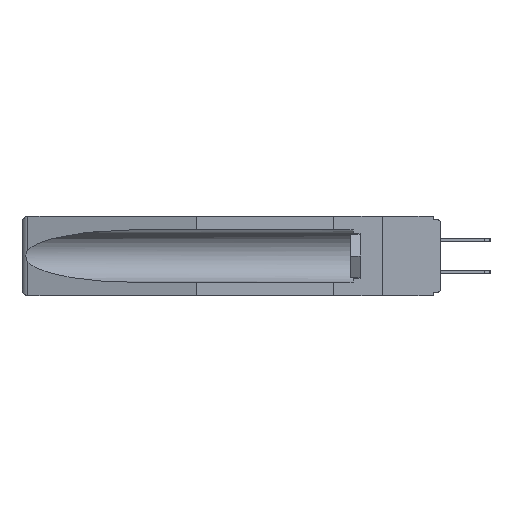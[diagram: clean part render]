
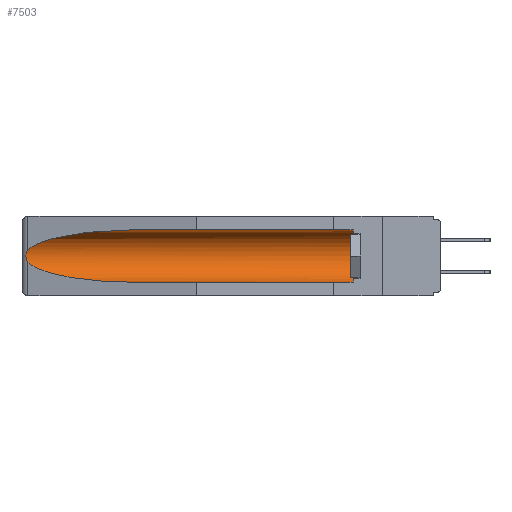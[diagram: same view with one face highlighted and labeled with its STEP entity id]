
A CAD part, left-side view. The second image highlights one B-rep face of the part: STEP entity #7503.
In plain terms, the highlighted cylindrical face has radius 2.857 mm (diameter 5.715 mm), a partial arc.
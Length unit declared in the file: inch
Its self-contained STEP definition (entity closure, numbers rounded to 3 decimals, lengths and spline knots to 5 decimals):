
#12 = CARTESIAN_POINT ( 'NONE',  ( 0.21114, 1.30732, -0.284 ) ) ;
#1002 = EDGE_LOOP ( 'NONE', ( #23991, #11615, #4133, #8195, #10715, #6035 ) ) ;
#1873 = AXIS2_PLACEMENT_3D ( 'NONE', #24452, #8560, #10771 ) ;
#2198 = CARTESIAN_POINT ( 'NONE',  ( 0.26597, 1.52961, -0.15275 ) ) ;
#2941 = CARTESIAN_POINT ( 'NONE',  ( 0.155, -0.30754, -0.284 ) ) ;
#4027 = VERTEX_POINT ( 'NONE', #26024 ) ;
#4091 = CARTESIAN_POINT ( 'NONE',  ( 0.155, 0.126, -0.284 ) ) ;
#4133 = ORIENTED_EDGE ( 'NONE', *, *, #19639, .T. ) ;
#5881 =( BOUNDED_CURVE ( )  B_SPLINE_CURVE ( 3, ( #20720, #25322, #7179, #11658 ),
 .UNSPECIFIED., .F., .F. ) 
 B_SPLINE_CURVE_WITH_KNOTS ( ( 4, 4 ),
 ( 4.71239, 6.08839 ),
 .UNSPECIFIED. ) 
 CURVE ( )  GEOMETRIC_REPRESENTATION_ITEM ( )  RATIONAL_B_SPLINE_CURVE ( ( 1., 0.848, 0.848, 1. ) ) 
 REPRESENTATION_ITEM ( '' )  );
#6035 = ORIENTED_EDGE ( 'NONE', *, *, #18235, .T. ) ;
#6184 = CARTESIAN_POINT ( 'NONE',  ( 0.155, 1.07973, -0.059 ) ) ;
#6787 = VERTEX_POINT ( 'NONE', #13449 ) ;
#6799 = CARTESIAN_POINT ( 'NONE',  ( 0.2675, 1.53308, -0.17534 ) ) ;
#6876 = LINE ( 'NONE', #10090, #29344 ) ;
#6960 = CIRCLE ( 'NONE', #1873, 0.1125 ) ;
#7024 = EDGE_CURVE ( 'NONE', #7655, #4027, #5881, .T. ) ;
#7094 = CARTESIAN_POINT ( 'NONE',  ( 0.26597, 1.5296, -0.19026 ) ) ;
#7179 = CARTESIAN_POINT ( 'NONE',  ( 0.25451, 1.48313, -0.09465 ) ) ;
#7503 = ADVANCED_FACE ( 'NONE', ( #28855 ), #17768, .F. ) ;
#7655 = VERTEX_POINT ( 'NONE', #6184 ) ;
#8195 = ORIENTED_EDGE ( 'NONE', *, *, #24356, .F. ) ;
#8560 = DIRECTION ( 'NONE',  ( 0., -1., 0. ) ) ;
#9345 = CARTESIAN_POINT ( 'NONE',  ( 0.26655, 1.53094, -0.18657 ) ) ;
#9802 = VERTEX_POINT ( 'NONE', #21206 ) ;
#10063 = VERTEX_POINT ( 'NONE', #24503 ) ;
#10090 = CARTESIAN_POINT ( 'NONE',  ( 0.155, -0.30754, -0.059 ) ) ;
#10715 = ORIENTED_EDGE ( 'NONE', *, *, #17072, .T. ) ;
#10771 = DIRECTION ( 'NONE',  ( 0., 0., 1. ) ) ;
#11158 = B_SPLINE_CURVE_WITH_KNOTS ( 'NONE', 3,
 ( #11564, #2198, #24940, #22628, #18446, #6799, #27322, #9345, #7094, #11269 ),
 .UNSPECIFIED., .F., .F.,
 ( 4, 2, 2, 2, 4 ),
 ( 0., 0.00029, 0.00058, 0.00087, 0.00117 ),
 .UNSPECIFIED. ) ;
#11269 = CARTESIAN_POINT ( 'NONE',  ( 0.26537, 1.52718, -0.19328 ) ) ;
#11564 = CARTESIAN_POINT ( 'NONE',  ( 0.26537, 1.52718, -0.14972 ) ) ;
#11615 = ORIENTED_EDGE ( 'NONE', *, *, #24021, .T. ) ;
#11658 = CARTESIAN_POINT ( 'NONE',  ( 0.26537, 1.52718, -0.14972 ) ) ;
#12024 = DIRECTION ( 'NONE',  ( 0., 1., 0. ) ) ;
#13449 = CARTESIAN_POINT ( 'NONE',  ( 0.155, 1.07973, -0.284 ) ) ;
#13534 =( BOUNDED_CURVE ( )  B_SPLINE_CURVE ( 3, ( #19833, #15449, #12, #17836 ),
 .UNSPECIFIED., .F., .F. ) 
 B_SPLINE_CURVE_WITH_KNOTS ( ( 4, 4 ),
 ( 0.1948, 1.5708 ),
 .UNSPECIFIED. ) 
 CURVE ( )  GEOMETRIC_REPRESENTATION_ITEM ( )  RATIONAL_B_SPLINE_CURVE ( ( 1., 0.848, 0.848, 1. ) ) 
 REPRESENTATION_ITEM ( '' )  );
#14046 = VERTEX_POINT ( 'NONE', #4091 ) ;
#14690 = DIRECTION ( 'NONE',  ( 0., 1., 0. ) ) ;
#14801 = VECTOR ( 'NONE', #12024, 39.37008 ) ;
#15449 = CARTESIAN_POINT ( 'NONE',  ( 0.25451, 1.48313, -0.24835 ) ) ;
#17072 = EDGE_CURVE ( 'NONE', #14046, #10063, #6960, .T. ) ;
#17768 = CYLINDRICAL_SURFACE ( 'NONE', #29103, 0.1125 ) ;
#17836 = CARTESIAN_POINT ( 'NONE',  ( 0.155, 1.07973, -0.284 ) ) ;
#18235 = EDGE_CURVE ( 'NONE', #10063, #7655, #6876, .T. ) ;
#18446 = CARTESIAN_POINT ( 'NONE',  ( 0.2675, 1.53308, -0.16763 ) ) ;
#19084 = DIRECTION ( 'NONE',  ( 0., 0., 1. ) ) ;
#19639 = EDGE_CURVE ( 'NONE', #9802, #6787, #13534, .T. ) ;
#19833 = CARTESIAN_POINT ( 'NONE',  ( 0.26537, 1.52718, -0.19328 ) ) ;
#20720 = CARTESIAN_POINT ( 'NONE',  ( 0.155, 1.07973, -0.059 ) ) ;
#21206 = CARTESIAN_POINT ( 'NONE',  ( 0.26537, 1.52718, -0.19328 ) ) ;
#22628 = CARTESIAN_POINT ( 'NONE',  ( 0.2673, 1.5327, -0.16383 ) ) ;
#23773 = DIRECTION ( 'NONE',  ( 0., 1., 0. ) ) ;
#23991 = ORIENTED_EDGE ( 'NONE', *, *, #7024, .T. ) ;
#24021 = EDGE_CURVE ( 'NONE', #4027, #9802, #11158, .T. ) ;
#24356 = EDGE_CURVE ( 'NONE', #14046, #6787, #24799, .T. ) ;
#24452 = CARTESIAN_POINT ( 'NONE',  ( 0.155, 0.126, -0.1715 ) ) ;
#24503 = CARTESIAN_POINT ( 'NONE',  ( 0.155, 0.126, -0.059 ) ) ;
#24799 = LINE ( 'NONE', #2941, #14801 ) ;
#24940 = CARTESIAN_POINT ( 'NONE',  ( 0.26654, 1.53092, -0.15636 ) ) ;
#25322 = CARTESIAN_POINT ( 'NONE',  ( 0.21114, 1.30732, -0.059 ) ) ;
#26024 = CARTESIAN_POINT ( 'NONE',  ( 0.26537, 1.52718, -0.14972 ) ) ;
#27322 = CARTESIAN_POINT ( 'NONE',  ( 0.2673, 1.53269, -0.17917 ) ) ;
#27641 = CARTESIAN_POINT ( 'NONE',  ( 0.155, -0.30754, -0.1715 ) ) ;
#28855 = FACE_OUTER_BOUND ( 'NONE', #1002, .T. ) ;
#29103 = AXIS2_PLACEMENT_3D ( 'NONE', #27641, #23773, #19084 ) ;
#29344 = VECTOR ( 'NONE', #14690, 39.37008 ) ;
